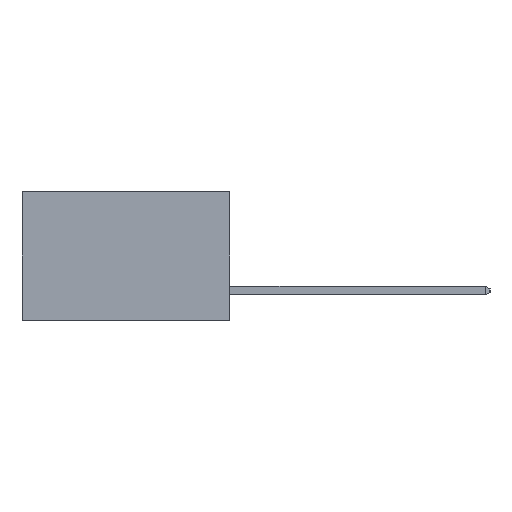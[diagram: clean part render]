
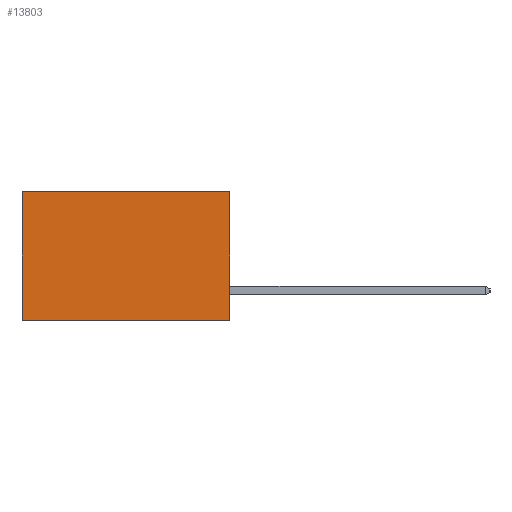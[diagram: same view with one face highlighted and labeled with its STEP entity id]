
A CAD part, left-side view. The second image highlights one B-rep face of the part: STEP entity #13803.
In plain terms, the highlighted planar face has unit normal (-1, 0, 0).
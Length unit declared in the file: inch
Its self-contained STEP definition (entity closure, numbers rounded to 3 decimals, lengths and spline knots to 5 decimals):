
#617 = VERTEX_POINT ( 'NONE', #28969 ) ;
#627 = CARTESIAN_POINT ( 'NONE',  ( 0.298, 0., 0. ) ) ;
#763 = AXIS2_PLACEMENT_3D ( 'NONE', #627, #18945, #5246 ) ;
#927 = VECTOR ( 'NONE', #21522, 39.37008 ) ;
#1022 = CARTESIAN_POINT ( 'NONE',  ( 0.298, 0., 0. ) ) ;
#1158 = CARTESIAN_POINT ( 'NONE',  ( 0.298, 0.6, -0.37 ) ) ;
#3242 = DIRECTION ( 'NONE',  ( 0., 0., -1. ) ) ;
#4502 = VERTEX_POINT ( 'NONE', #25861 ) ;
#5246 = DIRECTION ( 'NONE',  ( 0., 0., -1. ) ) ;
#6022 = VERTEX_POINT ( 'NONE', #9070 ) ;
#7028 = LINE ( 'NONE', #1022, #927 ) ;
#8598 = VECTOR ( 'NONE', #26253, 39.37008 ) ;
#8773 = DIRECTION ( 'NONE',  ( 0., 1., 0. ) ) ;
#9070 = CARTESIAN_POINT ( 'NONE',  ( 0.298, 0., -0.37 ) ) ;
#9259 = VECTOR ( 'NONE', #3242, 39.37008 ) ;
#9311 = LINE ( 'NONE', #23986, #8598 ) ;
#13567 = VECTOR ( 'NONE', #8773, 39.37008 ) ;
#13803 = ADVANCED_FACE ( 'NONE', ( #26757 ), #16614, .F. ) ;
#14567 = ORIENTED_EDGE ( 'NONE', *, *, #15759, .T. ) ;
#14596 = CARTESIAN_POINT ( 'NONE',  ( 0.298, 0.6, 0. ) ) ;
#15759 = EDGE_CURVE ( 'NONE', #617, #4502, #7028, .T. ) ;
#16058 = LINE ( 'NONE', #14596, #9259 ) ;
#16614 = PLANE ( 'NONE',  #763 ) ;
#17615 = VERTEX_POINT ( 'NONE', #1158 ) ;
#18183 = EDGE_CURVE ( 'NONE', #4502, #17615, #16058, .T. ) ;
#18945 = DIRECTION ( 'NONE',  ( 1., 0., 0. ) ) ;
#19066 = EDGE_LOOP ( 'NONE', ( #28929, #24147, #28908, #14567 ) ) ;
#21522 = DIRECTION ( 'NONE',  ( 0., 1., 0. ) ) ;
#22495 = CARTESIAN_POINT ( 'NONE',  ( 0.298, 0., -0.37 ) ) ;
#22915 = EDGE_CURVE ( 'NONE', #6022, #17615, #24344, .T. ) ;
#23986 = CARTESIAN_POINT ( 'NONE',  ( 0.298, 0., 0. ) ) ;
#24147 = ORIENTED_EDGE ( 'NONE', *, *, #22915, .F. ) ;
#24344 = LINE ( 'NONE', #22495, #13567 ) ;
#25861 = CARTESIAN_POINT ( 'NONE',  ( 0.298, 0.6, 0. ) ) ;
#26253 = DIRECTION ( 'NONE',  ( 0., 0., -1. ) ) ;
#26757 = FACE_OUTER_BOUND ( 'NONE', #19066, .T. ) ;
#28908 = ORIENTED_EDGE ( 'NONE', *, *, #29494, .F. ) ;
#28929 = ORIENTED_EDGE ( 'NONE', *, *, #18183, .T. ) ;
#28969 = CARTESIAN_POINT ( 'NONE',  ( 0.298, 0., 0. ) ) ;
#29494 = EDGE_CURVE ( 'NONE', #617, #6022, #9311, .T. ) ;
